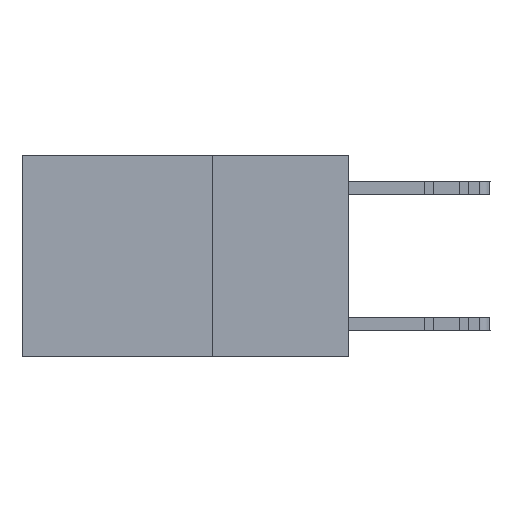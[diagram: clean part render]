
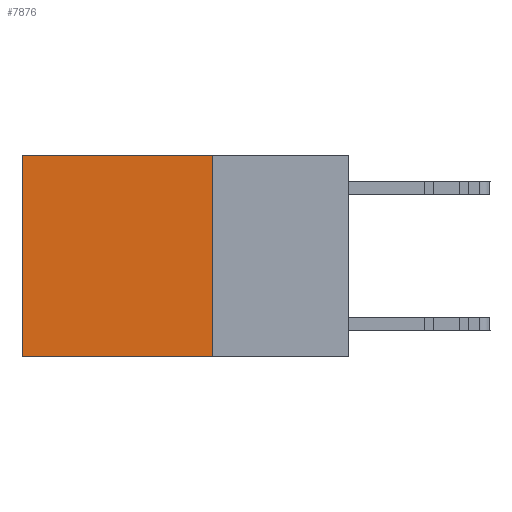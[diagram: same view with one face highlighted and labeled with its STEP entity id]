
A CAD part, left-side view. The second image highlights one B-rep face of the part: STEP entity #7876.
In plain terms, the highlighted planar face has unit normal (-1, 0, 0).
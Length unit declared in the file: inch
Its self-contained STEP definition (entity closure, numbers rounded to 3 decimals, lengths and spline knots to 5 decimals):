
#2298 = DIRECTION ( 'NONE',  ( 0., 1., 0. ) ) ;
#2621 = LINE ( 'NONE', #9492, #6904 ) ;
#3483 = CARTESIAN_POINT ( 'NONE',  ( 0.2625, 0.25, -0.37 ) ) ;
#6581 = AXIS2_PLACEMENT_3D ( 'NONE', #28913, #7125, #12368 ) ;
#6902 = DIRECTION ( 'NONE',  ( 0., 0., -1. ) ) ;
#6904 = VECTOR ( 'NONE', #2298, 39.37008 ) ;
#7125 = DIRECTION ( 'NONE',  ( 1., 0., 0. ) ) ;
#7581 = CARTESIAN_POINT ( 'NONE',  ( 0.2625, 0.25, -0.37 ) ) ;
#7594 = EDGE_CURVE ( 'NONE', #19803, #10814, #22000, .T. ) ;
#7876 = ADVANCED_FACE ( 'NONE', ( #9519 ), #19226, .F. ) ;
#8823 = EDGE_CURVE ( 'NONE', #12970, #10814, #14679, .T. ) ;
#9368 = ORIENTED_EDGE ( 'NONE', *, *, #12148, .T. ) ;
#9492 = CARTESIAN_POINT ( 'NONE',  ( 0.2625, 0.25, 0. ) ) ;
#9519 = FACE_OUTER_BOUND ( 'NONE', #17238, .T. ) ;
#9948 = CARTESIAN_POINT ( 'NONE',  ( 0.2625, 0.6, -0.37 ) ) ;
#10076 = ORIENTED_EDGE ( 'NONE', *, *, #8823, .T. ) ;
#10814 = VERTEX_POINT ( 'NONE', #9948 ) ;
#12108 = EDGE_CURVE ( 'NONE', #13532, #19803, #23974, .T. ) ;
#12148 = EDGE_CURVE ( 'NONE', #13532, #12970, #2621, .T. ) ;
#12368 = DIRECTION ( 'NONE',  ( 0., 0., -1. ) ) ;
#12712 = ORIENTED_EDGE ( 'NONE', *, *, #12108, .F. ) ;
#12970 = VERTEX_POINT ( 'NONE', #25807 ) ;
#13211 = DIRECTION ( 'NONE',  ( 0., 1., 0. ) ) ;
#13532 = VERTEX_POINT ( 'NONE', #18902 ) ;
#14533 = VECTOR ( 'NONE', #29741, 39.37008 ) ;
#14679 = LINE ( 'NONE', #29142, #14807 ) ;
#14807 = VECTOR ( 'NONE', #6902, 39.37008 ) ;
#17238 = EDGE_LOOP ( 'NONE', ( #10076, #21351, #12712, #9368 ) ) ;
#18902 = CARTESIAN_POINT ( 'NONE',  ( 0.2625, 0.25, 0. ) ) ;
#19226 = PLANE ( 'NONE',  #6581 ) ;
#19803 = VERTEX_POINT ( 'NONE', #7581 ) ;
#21351 = ORIENTED_EDGE ( 'NONE', *, *, #7594, .F. ) ;
#21746 = CARTESIAN_POINT ( 'NONE',  ( 0.2625, 0.25, 0. ) ) ;
#22000 = LINE ( 'NONE', #3483, #23342 ) ;
#23342 = VECTOR ( 'NONE', #13211, 39.37008 ) ;
#23974 = LINE ( 'NONE', #21746, #14533 ) ;
#25807 = CARTESIAN_POINT ( 'NONE',  ( 0.2625, 0.6, 0. ) ) ;
#28913 = CARTESIAN_POINT ( 'NONE',  ( 0.2625, 0.25, 0. ) ) ;
#29142 = CARTESIAN_POINT ( 'NONE',  ( 0.2625, 0.6, 0. ) ) ;
#29741 = DIRECTION ( 'NONE',  ( 0., 0., -1. ) ) ;
